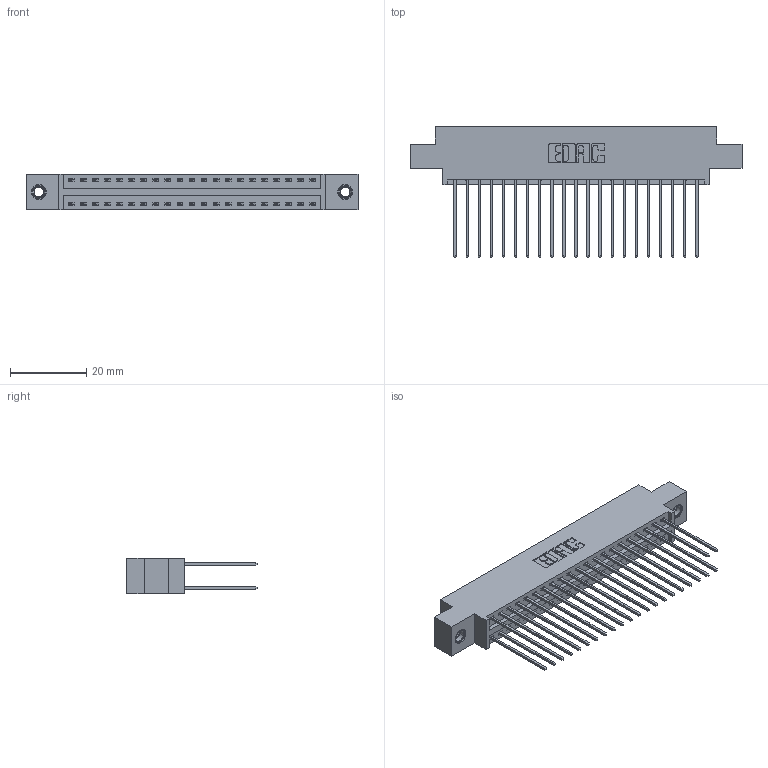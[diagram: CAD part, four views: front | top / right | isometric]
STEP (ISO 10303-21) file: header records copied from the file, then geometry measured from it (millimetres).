
FILE_DESCRIPTION (( 'STEP AP203' ), '1' );
FILE_NAME ('346-042-541-807.STEP', '2022-05-20T04:47:25', ( '' ), ( '' ), 'SwSTEP 2.0', 'SolidWorks 2020', '' );
FILE_SCHEMA (( 'CONFIG_CONTROL_DESIGN' ));
Length unit declared in the file: inch
Products named in the file (4): 346 Part_0.170 Offset - 0.156 Dia-TI; 345-292-001_345-293-141; 345-250-001_345-250-005-103; 346-042-541-807
Assembly tree (45 placements, depth 2):
  346-042-541-807
    346 Part_0.170 Offset - 0.156 Dia-TI
    345-292-001_345-293-141  x42
    345-250-001_345-250-005-103  x2
Bounding box: 87.25 x 34.29 x 9.4 mm (x, y, z)
Volume: 8417.6 mm3; surface area: 12609.4 mm2
Topology: 45 solids, 45 shells, 2370 faces, 6987 edges, 4594 vertices
Faces by surface type: plane 1582, cylinder 772, cone 12, torus 4
Entity records: 17868 total; most frequent: CARTESIAN_POINT 2959, ORIENTED_EDGE 2886, DIRECTION 2685, EDGE_CURVE 1443, LINE 1207, VECTOR 1207, VERTEX_POINT 956, AXIS2_PLACEMENT_3D 739
